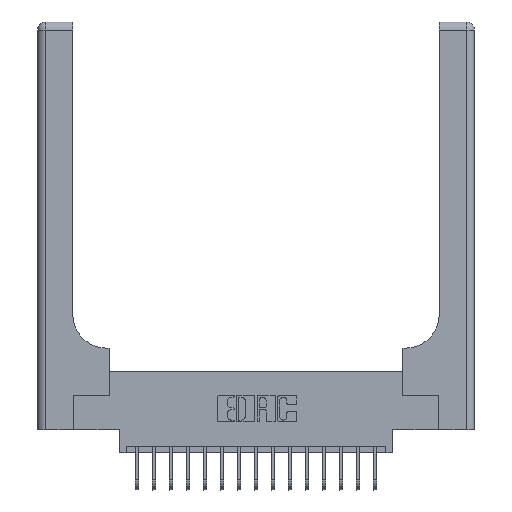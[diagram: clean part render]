
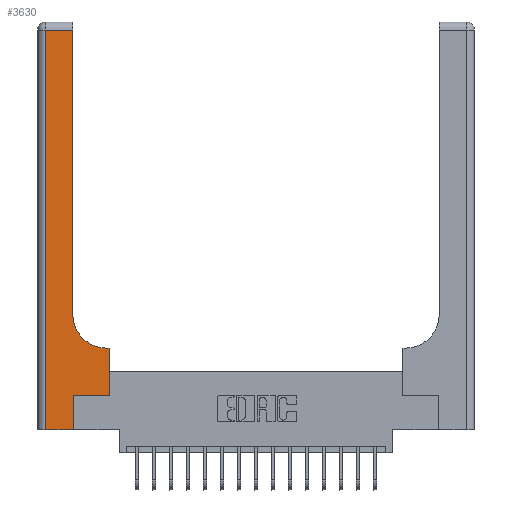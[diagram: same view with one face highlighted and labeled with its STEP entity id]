
A CAD part, top view. The second image highlights one B-rep face of the part: STEP entity #3630.
In plain terms, the highlighted planar face has unit normal (0, 0, 1).
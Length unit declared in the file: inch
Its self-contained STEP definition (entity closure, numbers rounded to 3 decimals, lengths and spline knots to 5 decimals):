
#114 = DIRECTION ( 'NONE',  ( 0., 1., 0. ) ) ;
#383 = CARTESIAN_POINT ( 'NONE',  ( 0.26, 0.6, 0.37 ) ) ;
#402 = CARTESIAN_POINT ( 'NONE',  ( 0.528, 0.25, 0.37 ) ) ;
#589 = ORIENTED_EDGE ( 'NONE', *, *, #10555, .T. ) ;
#820 = LINE ( 'NONE', #2097, #20143 ) ;
#1143 = VERTEX_POINT ( 'NONE', #6583 ) ;
#1234 = EDGE_CURVE ( 'NONE', #1812, #18590, #13800, .T. ) ;
#1739 = ORIENTED_EDGE ( 'NONE', *, *, #15514, .T. ) ;
#1812 = VERTEX_POINT ( 'NONE', #4689 ) ;
#2097 = CARTESIAN_POINT ( 'NONE',  ( 0.265, 0.25, 0.37 ) ) ;
#2448 = VERTEX_POINT ( 'NONE', #20371 ) ;
#2722 = CARTESIAN_POINT ( 'NONE',  ( 0.26, 3., 0.37 ) ) ;
#3055 = LINE ( 'NONE', #14807, #13213 ) ;
#3398 = EDGE_CURVE ( 'NONE', #1143, #2448, #19962, .T. ) ;
#3536 = FACE_OUTER_BOUND ( 'NONE', #14196, .T. ) ;
#3570 = ORIENTED_EDGE ( 'NONE', *, *, #12898, .T. ) ;
#3630 = ADVANCED_FACE ( 'NONE', ( #3536 ), #5315, .F. ) ;
#4007 = DIRECTION ( 'NONE',  ( 0., 1., 0. ) ) ;
#4230 = CARTESIAN_POINT ( 'NONE',  ( 0.51, 0.85, 0.37 ) ) ;
#4689 = CARTESIAN_POINT ( 'NONE',  ( 0.51, 0.6, 0.37 ) ) ;
#5219 = DIRECTION ( 'NONE',  ( 0., 0., -1. ) ) ;
#5315 = PLANE ( 'NONE',  #14639 ) ;
#5992 = CARTESIAN_POINT ( 'NONE',  ( 0.265, 0., 0.37 ) ) ;
#6359 = CARTESIAN_POINT ( 'NONE',  ( 0.06, 3., 0.37 ) ) ;
#6583 = CARTESIAN_POINT ( 'NONE',  ( 0.26, 2.94, 0.37 ) ) ;
#6695 = ORIENTED_EDGE ( 'NONE', *, *, #14718, .T. ) ;
#6815 = DIRECTION ( 'NONE',  ( -1., 0., 0. ) ) ;
#6948 = DIRECTION ( 'NONE',  ( 1., 0., 0. ) ) ;
#8158 = LINE ( 'NONE', #6359, #13296 ) ;
#8696 = DIRECTION ( 'NONE',  ( 0., 0., -1. ) ) ;
#8818 = VECTOR ( 'NONE', #13645, 39.37008 ) ;
#9666 = VERTEX_POINT ( 'NONE', #16177 ) ;
#9765 = ORIENTED_EDGE ( 'NONE', *, *, #12981, .T. ) ;
#10141 = LINE ( 'NONE', #383, #8818 ) ;
#10277 = CARTESIAN_POINT ( 'NONE',  ( 0.06, 0., 0.37 ) ) ;
#10555 = EDGE_CURVE ( 'NONE', #18590, #1143, #12170, .T. ) ;
#11378 = VERTEX_POINT ( 'NONE', #10277 ) ;
#11476 = CARTESIAN_POINT ( 'NONE',  ( 0.528, 0.25, 0.37 ) ) ;
#11693 = ORIENTED_EDGE ( 'NONE', *, *, #19795, .T. ) ;
#11799 = DIRECTION ( 'NONE',  ( -1., 0., 0. ) ) ;
#11927 = LINE ( 'NONE', #18403, #16311 ) ;
#12103 = EDGE_CURVE ( 'NONE', #19368, #17502, #14757, .T. ) ;
#12160 = DIRECTION ( 'NONE',  ( 1., 0., 0. ) ) ;
#12170 = LINE ( 'NONE', #2722, #13494 ) ;
#12898 = EDGE_CURVE ( 'NONE', #18975, #9666, #3055, .T. ) ;
#12981 = EDGE_CURVE ( 'NONE', #17502, #1812, #10141, .T. ) ;
#13122 = DIRECTION ( 'NONE',  ( 0., 1., 0. ) ) ;
#13213 = VECTOR ( 'NONE', #13122, 39.37008 ) ;
#13296 = VECTOR ( 'NONE', #19733, 39.37008 ) ;
#13494 = VECTOR ( 'NONE', #4007, 39.37008 ) ;
#13645 = DIRECTION ( 'NONE',  ( -1., 0., 0. ) ) ;
#13800 = CIRCLE ( 'NONE', #16845, 0.25 ) ;
#14196 = EDGE_LOOP ( 'NONE', ( #589, #19726, #1739, #6695, #3570, #11693, #18044, #9765, #19786 ) ) ;
#14639 = AXIS2_PLACEMENT_3D ( 'NONE', #19658, #5219, #11799 ) ;
#14718 = EDGE_CURVE ( 'NONE', #11378, #18975, #11927, .T. ) ;
#14757 = LINE ( 'NONE', #11476, #15202 ) ;
#14807 = CARTESIAN_POINT ( 'NONE',  ( 0.265, 0., 0.37 ) ) ;
#15202 = VECTOR ( 'NONE', #114, 39.37008 ) ;
#15334 = CARTESIAN_POINT ( 'NONE',  ( 0.528, 0.6, 0.37 ) ) ;
#15514 = EDGE_CURVE ( 'NONE', #2448, #11378, #8158, .T. ) ;
#16177 = CARTESIAN_POINT ( 'NONE',  ( 0.265, 0.25, 0.37 ) ) ;
#16311 = VECTOR ( 'NONE', #6948, 39.37008 ) ;
#16845 = AXIS2_PLACEMENT_3D ( 'NONE', #4230, #8696, #20259 ) ;
#17502 = VERTEX_POINT ( 'NONE', #15334 ) ;
#17963 = CARTESIAN_POINT ( 'NONE',  ( 0., 2.94, 0.37 ) ) ;
#18010 = CARTESIAN_POINT ( 'NONE',  ( 0.26, 0.85, 0.37 ) ) ;
#18044 = ORIENTED_EDGE ( 'NONE', *, *, #12103, .T. ) ;
#18381 = VECTOR ( 'NONE', #6815, 39.37008 ) ;
#18403 = CARTESIAN_POINT ( 'NONE',  ( 0., 0., 0.37 ) ) ;
#18590 = VERTEX_POINT ( 'NONE', #18010 ) ;
#18975 = VERTEX_POINT ( 'NONE', #5992 ) ;
#19368 = VERTEX_POINT ( 'NONE', #402 ) ;
#19658 = CARTESIAN_POINT ( 'NONE',  ( 0., 3., 0.37 ) ) ;
#19726 = ORIENTED_EDGE ( 'NONE', *, *, #3398, .T. ) ;
#19733 = DIRECTION ( 'NONE',  ( 0., -1., 0. ) ) ;
#19786 = ORIENTED_EDGE ( 'NONE', *, *, #1234, .T. ) ;
#19795 = EDGE_CURVE ( 'NONE', #9666, #19368, #820, .T. ) ;
#19962 = LINE ( 'NONE', #17963, #18381 ) ;
#20143 = VECTOR ( 'NONE', #12160, 39.37008 ) ;
#20259 = DIRECTION ( 'NONE',  ( 1., 0., 0. ) ) ;
#20371 = CARTESIAN_POINT ( 'NONE',  ( 0.06, 2.94, 0.37 ) ) ;
